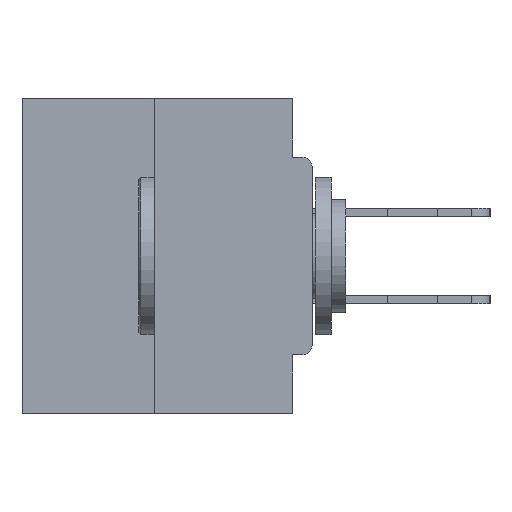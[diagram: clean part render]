
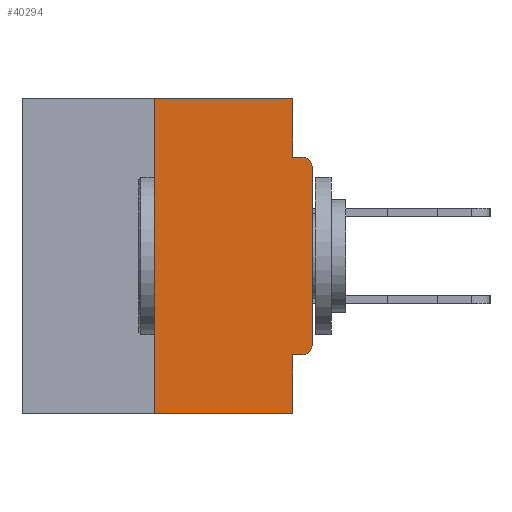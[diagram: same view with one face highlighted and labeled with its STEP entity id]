
A CAD part, left-side view. The second image highlights one B-rep face of the part: STEP entity #40294.
In plain terms, the highlighted planar face has unit normal (-1, 0, 0).
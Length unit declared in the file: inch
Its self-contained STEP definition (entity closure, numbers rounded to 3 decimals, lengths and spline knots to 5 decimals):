
#34 = CARTESIAN_POINT ( 'NONE',  ( 0., 0.015, -0.1085 ) ) ;
#453 = EDGE_CURVE ( 'NONE', #15122, #17611, #33431, .T. ) ;
#724 = VECTOR ( 'NONE', #6061, 39.37008 ) ;
#909 = CARTESIAN_POINT ( 'NONE',  ( 0., 0.031, -0.5 ) ) ;
#979 = VERTEX_POINT ( 'NONE', #7355 ) ;
#1053 = EDGE_CURVE ( 'NONE', #35266, #12541, #21294, .T. ) ;
#1111 = ORIENTED_EDGE ( 'NONE', *, *, #14025, .T. ) ;
#2182 = CARTESIAN_POINT ( 'NONE',  ( 0., 0.031, 0. ) ) ;
#2612 = EDGE_CURVE ( 'NONE', #42683, #32242, #22183, .T. ) ;
#3698 = DIRECTION ( 'NONE',  ( 0., 0., -1. ) ) ;
#6061 = DIRECTION ( 'NONE',  ( 0., -1., 0. ) ) ;
#6339 = ORIENTED_EDGE ( 'NONE', *, *, #2612, .F. ) ;
#7325 = EDGE_CURVE ( 'NONE', #979, #40309, #40903, .T. ) ;
#7355 = CARTESIAN_POINT ( 'NONE',  ( 0., 0.25, -0.5 ) ) ;
#7924 = DIRECTION ( 'NONE',  ( 0., 0., 1. ) ) ;
#7984 = FACE_OUTER_BOUND ( 'NONE', #20833, .T. ) ;
#8033 = ORIENTED_EDGE ( 'NONE', *, *, #25336, .F. ) ;
#9010 = ORIENTED_EDGE ( 'NONE', *, *, #7325, .T. ) ;
#9394 = CARTESIAN_POINT ( 'NONE',  ( 0., 0.031, -0.4065 ) ) ;
#9528 = LINE ( 'NONE', #12911, #10095 ) ;
#9687 = CARTESIAN_POINT ( 'NONE',  ( 0., 0.015, -0.4065 ) ) ;
#10095 = VECTOR ( 'NONE', #32887, 39.37008 ) ;
#10217 = DIRECTION ( 'NONE',  ( 0., -1., 0. ) ) ;
#10376 = CARTESIAN_POINT ( 'NONE',  ( 0., 0.25, 0. ) ) ;
#11572 = CARTESIAN_POINT ( 'NONE',  ( 0., 0.031, -0.0935 ) ) ;
#12541 = VERTEX_POINT ( 'NONE', #39933 ) ;
#12744 = DIRECTION ( 'NONE',  ( -1., 0., 0. ) ) ;
#12911 = CARTESIAN_POINT ( 'NONE',  ( 0., 0.25, 0. ) ) ;
#12947 = LINE ( 'NONE', #15720, #724 ) ;
#13754 = EDGE_CURVE ( 'NONE', #35420, #42683, #25246, .T. ) ;
#14015 = VECTOR ( 'NONE', #31463, 39.37008 ) ;
#14025 = EDGE_CURVE ( 'NONE', #12541, #36195, #36839, .T. ) ;
#15122 = VERTEX_POINT ( 'NONE', #9687 ) ;
#15720 = CARTESIAN_POINT ( 'NONE',  ( 0., 0., -0.0935 ) ) ;
#17167 = EDGE_CURVE ( 'NONE', #15122, #35266, #37555, .T. ) ;
#17427 = CARTESIAN_POINT ( 'NONE',  ( 0., 0.46, -0.5 ) ) ;
#17611 = VERTEX_POINT ( 'NONE', #9394 ) ;
#17775 = VECTOR ( 'NONE', #10217, 39.37008 ) ;
#17939 = DIRECTION ( 'NONE',  ( 0., 0., -1. ) ) ;
#17967 = CARTESIAN_POINT ( 'NONE',  ( 0., 0., 0. ) ) ;
#18086 = DIRECTION ( 'NONE',  ( 1., 0., 0. ) ) ;
#18094 = AXIS2_PLACEMENT_3D ( 'NONE', #34, #36917, #3698 ) ;
#18164 = VECTOR ( 'NONE', #37181, 39.37008 ) ;
#18213 = ORIENTED_EDGE ( 'NONE', *, *, #453, .F. ) ;
#19458 = CARTESIAN_POINT ( 'NONE',  ( 0., 0.46, 0. ) ) ;
#20833 = EDGE_LOOP ( 'NONE', ( #39096, #41461, #9010, #8033, #18213, #27714, #24555, #1111, #38696, #6339 ) ) ;
#21229 = CARTESIAN_POINT ( 'NONE',  ( 0., 0.031, 0. ) ) ;
#21294 = LINE ( 'NONE', #17967, #36006 ) ;
#21353 = CARTESIAN_POINT ( 'NONE',  ( 0., 0.46, 0. ) ) ;
#21880 = CARTESIAN_POINT ( 'NONE',  ( 0., 0.015, -0.0935 ) ) ;
#22183 = LINE ( 'NONE', #2182, #42663 ) ;
#24555 = ORIENTED_EDGE ( 'NONE', *, *, #1053, .T. ) ;
#25246 = LINE ( 'NONE', #19458, #38381 ) ;
#25336 = EDGE_CURVE ( 'NONE', #17611, #40309, #30867, .T. ) ;
#25578 = EDGE_CURVE ( 'NONE', #32242, #36195, #12947, .T. ) ;
#26147 = DIRECTION ( 'NONE',  ( 0., 0., -1. ) ) ;
#27528 = CARTESIAN_POINT ( 'NONE',  ( 0., 0.031, -0.5 ) ) ;
#27714 = ORIENTED_EDGE ( 'NONE', *, *, #17167, .T. ) ;
#27826 = PLANE ( 'NONE',  #31947 ) ;
#30867 = LINE ( 'NONE', #909, #14015 ) ;
#31463 = DIRECTION ( 'NONE',  ( 0., 0., -1. ) ) ;
#31947 = AXIS2_PLACEMENT_3D ( 'NONE', #21353, #18086, #17939 ) ;
#32242 = VERTEX_POINT ( 'NONE', #11572 ) ;
#32887 = DIRECTION ( 'NONE',  ( 0., 0., 1. ) ) ;
#33112 = DIRECTION ( 'NONE',  ( 0., -1., 0. ) ) ;
#33431 = LINE ( 'NONE', #33755, #18164 ) ;
#33755 = CARTESIAN_POINT ( 'NONE',  ( 0., 0., -0.4065 ) ) ;
#35266 = VERTEX_POINT ( 'NONE', #35967 ) ;
#35338 = AXIS2_PLACEMENT_3D ( 'NONE', #40895, #12744, #39969 ) ;
#35420 = VERTEX_POINT ( 'NONE', #10376 ) ;
#35967 = CARTESIAN_POINT ( 'NONE',  ( 0., 0., -0.3915 ) ) ;
#36006 = VECTOR ( 'NONE', #7924, 39.37008 ) ;
#36195 = VERTEX_POINT ( 'NONE', #21880 ) ;
#36839 = CIRCLE ( 'NONE', #18094, 0.015 ) ;
#36917 = DIRECTION ( 'NONE',  ( -1., 0., 0. ) ) ;
#37181 = DIRECTION ( 'NONE',  ( 0., 1., 0. ) ) ;
#37555 = CIRCLE ( 'NONE', #35338, 0.015 ) ;
#38381 = VECTOR ( 'NONE', #33112, 39.37008 ) ;
#38696 = ORIENTED_EDGE ( 'NONE', *, *, #25578, .F. ) ;
#39096 = ORIENTED_EDGE ( 'NONE', *, *, #13754, .F. ) ;
#39933 = CARTESIAN_POINT ( 'NONE',  ( 0., 0., -0.1085 ) ) ;
#39969 = DIRECTION ( 'NONE',  ( 0., 0., -1. ) ) ;
#40294 = ADVANCED_FACE ( 'NONE', ( #7984 ), #27826, .F. ) ;
#40309 = VERTEX_POINT ( 'NONE', #27528 ) ;
#40895 = CARTESIAN_POINT ( 'NONE',  ( 0., 0.015, -0.3915 ) ) ;
#40903 = LINE ( 'NONE', #17427, #17775 ) ;
#41039 = EDGE_CURVE ( 'NONE', #979, #35420, #9528, .T. ) ;
#41461 = ORIENTED_EDGE ( 'NONE', *, *, #41039, .F. ) ;
#42663 = VECTOR ( 'NONE', #26147, 39.37008 ) ;
#42683 = VERTEX_POINT ( 'NONE', #21229 ) ;
